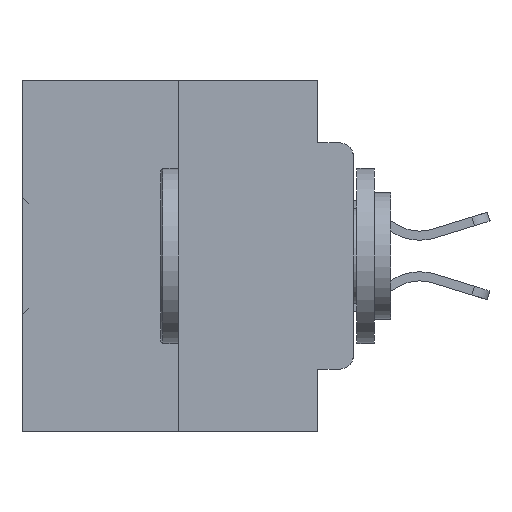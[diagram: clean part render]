
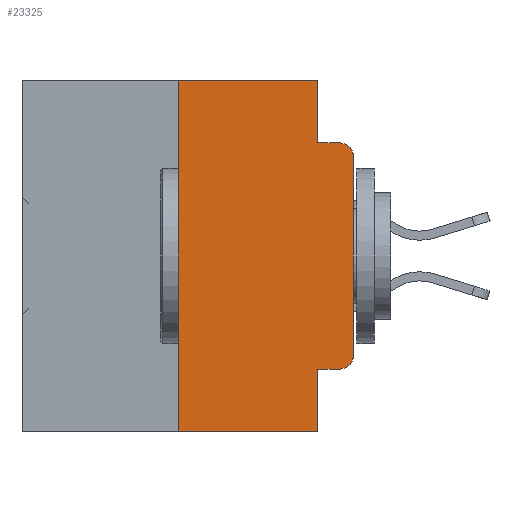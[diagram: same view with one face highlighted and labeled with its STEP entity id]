
A CAD part, left-side view. The second image highlights one B-rep face of the part: STEP entity #23325.
In plain terms, the highlighted planar face has unit normal (-1, 0, 0).
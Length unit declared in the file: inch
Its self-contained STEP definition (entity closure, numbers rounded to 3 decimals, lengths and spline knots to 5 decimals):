
#774 = VECTOR ( 'NONE', #34731, 39.37008 ) ;
#1459 = VECTOR ( 'NONE', #11903, 39.37008 ) ;
#1570 = EDGE_CURVE ( 'NONE', #5392, #25577, #13748, .T. ) ;
#1818 = VECTOR ( 'NONE', #16906, 39.37008 ) ;
#2172 = CARTESIAN_POINT ( 'NONE',  ( 0., 0.051, 0. ) ) ;
#2430 = CARTESIAN_POINT ( 'NONE',  ( 0., 0.051, -0.4115 ) ) ;
#2511 = DIRECTION ( 'NONE',  ( 0., 0., -1. ) ) ;
#2931 = CARTESIAN_POINT ( 'NONE',  ( 0., 0.051, -0.0885 ) ) ;
#3145 = VERTEX_POINT ( 'NONE', #27703 ) ;
#3228 = CARTESIAN_POINT ( 'NONE',  ( 0., 0.02, -0.1085 ) ) ;
#4296 = DIRECTION ( 'NONE',  ( 0., -1., 0. ) ) ;
#5366 = PLANE ( 'NONE',  #13570 ) ;
#5392 = VERTEX_POINT ( 'NONE', #9629 ) ;
#5970 = CARTESIAN_POINT ( 'NONE',  ( 0., 0.051, 0. ) ) ;
#6278 = CARTESIAN_POINT ( 'NONE',  ( 0., 0.02, -0.3915 ) ) ;
#6712 = ORIENTED_EDGE ( 'NONE', *, *, #18928, .T. ) ;
#7499 = VERTEX_POINT ( 'NONE', #2172 ) ;
#7660 = DIRECTION ( 'NONE',  ( 0., 0., -1. ) ) ;
#8226 = FACE_OUTER_BOUND ( 'NONE', #27860, .T. ) ;
#9629 = CARTESIAN_POINT ( 'NONE',  ( 0., 0., -0.3915 ) ) ;
#9931 = VECTOR ( 'NONE', #18018, 39.37008 ) ;
#10147 = ORIENTED_EDGE ( 'NONE', *, *, #33331, .F. ) ;
#10163 = VECTOR ( 'NONE', #33864, 39.37008 ) ;
#10208 = VECTOR ( 'NONE', #7660, 39.37008 ) ;
#10536 = CARTESIAN_POINT ( 'NONE',  ( 0., 0.051, 0. ) ) ;
#11339 = CARTESIAN_POINT ( 'NONE',  ( 0., 0.02, -0.4115 ) ) ;
#11903 = DIRECTION ( 'NONE',  ( 0., 0., 1. ) ) ;
#12025 = DIRECTION ( 'NONE',  ( -1., 0., 0. ) ) ;
#12217 = DIRECTION ( 'NONE',  ( 0., 0., -1. ) ) ;
#12394 = VECTOR ( 'NONE', #15360, 39.37008 ) ;
#13057 = ORIENTED_EDGE ( 'NONE', *, *, #14420, .T. ) ;
#13187 = AXIS2_PLACEMENT_3D ( 'NONE', #3228, #12025, #12217 ) ;
#13570 = AXIS2_PLACEMENT_3D ( 'NONE', #17028, #28697, #2511 ) ;
#13748 = LINE ( 'NONE', #25430, #10163 ) ;
#14238 = EDGE_CURVE ( 'NONE', #3145, #37662, #36752, .T. ) ;
#14420 = EDGE_CURVE ( 'NONE', #34559, #5392, #35864, .T. ) ;
#14697 = EDGE_CURVE ( 'NONE', #24142, #25799, #37176, .T. ) ;
#14773 = LINE ( 'NONE', #26442, #1459 ) ;
#14971 = LINE ( 'NONE', #27026, #12394 ) ;
#15105 = DIRECTION ( 'NONE',  ( 0., 0., -1. ) ) ;
#15360 = DIRECTION ( 'NONE',  ( 0., -1., 0. ) ) ;
#15496 = ORIENTED_EDGE ( 'NONE', *, *, #24155, .F. ) ;
#15624 = ORIENTED_EDGE ( 'NONE', *, *, #24237, .F. ) ;
#15742 = VECTOR ( 'NONE', #4296, 39.37008 ) ;
#16536 = LINE ( 'NONE', #34328, #1818 ) ;
#16906 = DIRECTION ( 'NONE',  ( 0., -1., 0. ) ) ;
#17028 = CARTESIAN_POINT ( 'NONE',  ( 0., 0.473, 0. ) ) ;
#18018 = DIRECTION ( 'NONE',  ( 0., 0., -1. ) ) ;
#18560 = CARTESIAN_POINT ( 'NONE',  ( 0., 0.25, -0.5 ) ) ;
#18853 = VERTEX_POINT ( 'NONE', #31448 ) ;
#18928 = EDGE_CURVE ( 'NONE', #35365, #37662, #16536, .T. ) ;
#19361 = AXIS2_PLACEMENT_3D ( 'NONE', #6278, #29824, #15105 ) ;
#20739 = CARTESIAN_POINT ( 'NONE',  ( 0., 0., -0.1085 ) ) ;
#20768 = ORIENTED_EDGE ( 'NONE', *, *, #30652, .T. ) ;
#22118 = ORIENTED_EDGE ( 'NONE', *, *, #14238, .F. ) ;
#22611 = CARTESIAN_POINT ( 'NONE',  ( 0., 0.051, -0.5 ) ) ;
#23325 = ADVANCED_FACE ( 'NONE', ( #8226 ), #5366, .F. ) ;
#24142 = VERTEX_POINT ( 'NONE', #2931 ) ;
#24155 = EDGE_CURVE ( 'NONE', #7499, #24142, #32182, .T. ) ;
#24237 = EDGE_CURVE ( 'NONE', #18853, #7499, #14971, .T. ) ;
#24804 = CIRCLE ( 'NONE', #13187, 0.02 ) ;
#25430 = CARTESIAN_POINT ( 'NONE',  ( 0., 0., 0. ) ) ;
#25577 = VERTEX_POINT ( 'NONE', #20739 ) ;
#25799 = VERTEX_POINT ( 'NONE', #35390 ) ;
#25974 = ORIENTED_EDGE ( 'NONE', *, *, #1570, .T. ) ;
#26442 = CARTESIAN_POINT ( 'NONE',  ( 0., 0.25, 0. ) ) ;
#27026 = CARTESIAN_POINT ( 'NONE',  ( 0., 0.473, 0. ) ) ;
#27382 = EDGE_CURVE ( 'NONE', #25577, #25799, #24804, .T. ) ;
#27703 = CARTESIAN_POINT ( 'NONE',  ( 0., 0.051, -0.4115 ) ) ;
#27860 = EDGE_LOOP ( 'NONE', ( #25974, #36397, #32399, #15496, #15624, #10147, #6712, #22118, #20768, #13057 ) ) ;
#28697 = DIRECTION ( 'NONE',  ( 1., 0., 0. ) ) ;
#29824 = DIRECTION ( 'NONE',  ( -1., 0., 0. ) ) ;
#30652 = EDGE_CURVE ( 'NONE', #3145, #34559, #30929, .T. ) ;
#30929 = LINE ( 'NONE', #2430, #774 ) ;
#31448 = CARTESIAN_POINT ( 'NONE',  ( 0., 0.25, 0. ) ) ;
#32182 = LINE ( 'NONE', #5970, #9931 ) ;
#32399 = ORIENTED_EDGE ( 'NONE', *, *, #14697, .F. ) ;
#33331 = EDGE_CURVE ( 'NONE', #35365, #18853, #14773, .T. ) ;
#33864 = DIRECTION ( 'NONE',  ( 0., 0., 1. ) ) ;
#34310 = CARTESIAN_POINT ( 'NONE',  ( 0., 0.051, -0.0885 ) ) ;
#34328 = CARTESIAN_POINT ( 'NONE',  ( 0., 0.473, -0.5 ) ) ;
#34559 = VERTEX_POINT ( 'NONE', #11339 ) ;
#34731 = DIRECTION ( 'NONE',  ( 0., -1., 0. ) ) ;
#35365 = VERTEX_POINT ( 'NONE', #18560 ) ;
#35390 = CARTESIAN_POINT ( 'NONE',  ( 0., 0.02, -0.0885 ) ) ;
#35864 = CIRCLE ( 'NONE', #19361, 0.02 ) ;
#36397 = ORIENTED_EDGE ( 'NONE', *, *, #27382, .T. ) ;
#36752 = LINE ( 'NONE', #10536, #10208 ) ;
#37176 = LINE ( 'NONE', #34310, #15742 ) ;
#37662 = VERTEX_POINT ( 'NONE', #22611 ) ;
